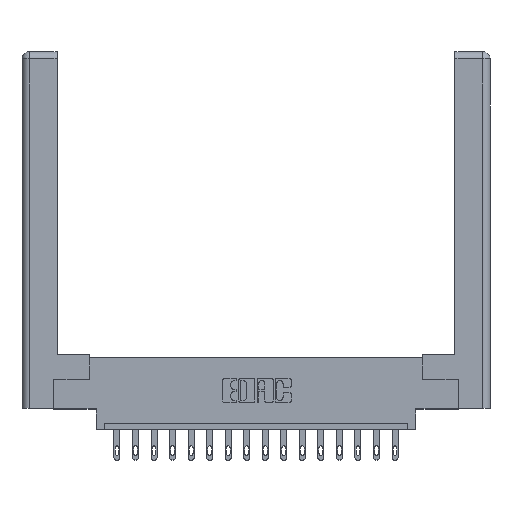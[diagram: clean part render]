
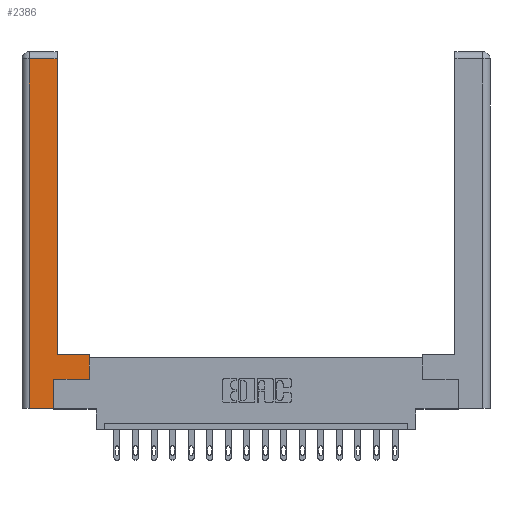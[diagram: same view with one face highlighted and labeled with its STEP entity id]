
A CAD part, top view. The second image highlights one B-rep face of the part: STEP entity #2386.
In plain terms, the highlighted planar face has unit normal (0, 0, 1).
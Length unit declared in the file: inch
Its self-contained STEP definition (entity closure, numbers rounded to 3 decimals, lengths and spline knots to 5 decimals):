
#383 = CARTESIAN_POINT ( 'NONE',  ( 0.565, 0.45, 0. ) ) ;
#586 = VERTEX_POINT ( 'NONE', #3452 ) ;
#649 = CARTESIAN_POINT ( 'NONE',  ( 0.265, 0.245, 0. ) ) ;
#767 = CARTESIAN_POINT ( 'NONE',  ( 0.265, 0.245, 0. ) ) ;
#811 = ORIENTED_EDGE ( 'NONE', *, *, #1996, .T. ) ;
#1185 = CARTESIAN_POINT ( 'NONE',  ( 0.0615, 2.94, 0. ) ) ;
#1255 = VERTEX_POINT ( 'NONE', #9296 ) ;
#1418 = LINE ( 'NONE', #2562, #4699 ) ;
#1996 = EDGE_CURVE ( 'NONE', #586, #2529, #3529, .T. ) ;
#2221 = EDGE_CURVE ( 'NONE', #3925, #12713, #11321, .T. ) ;
#2386 = ADVANCED_FACE ( 'NONE', ( #11115 ), #7721, .F. ) ;
#2529 = VERTEX_POINT ( 'NONE', #13905 ) ;
#2562 = CARTESIAN_POINT ( 'NONE',  ( 0.265, 0., 0. ) ) ;
#2714 = CARTESIAN_POINT ( 'NONE',  ( 0.295, 3., 0. ) ) ;
#2833 = VECTOR ( 'NONE', #14444, 39.37008 ) ;
#3452 = CARTESIAN_POINT ( 'NONE',  ( 0.565, 0.245, 0. ) ) ;
#3529 = LINE ( 'NONE', #383, #3743 ) ;
#3743 = VECTOR ( 'NONE', #8595, 39.37008 ) ;
#3925 = VERTEX_POINT ( 'NONE', #11253 ) ;
#4699 = VECTOR ( 'NONE', #16469, 39.37008 ) ;
#4761 = DIRECTION ( 'NONE',  ( 0., 0., -1. ) ) ;
#5223 = LINE ( 'NONE', #767, #2833 ) ;
#5252 = VECTOR ( 'NONE', #15096, 39.37008 ) ;
#5831 = CARTESIAN_POINT ( 'NONE',  ( 0.565, 0.245, 0. ) ) ;
#6447 = EDGE_LOOP ( 'NONE', ( #8512, #17109, #12081, #16028, #7685, #17517, #811, #10173 ) ) ;
#6789 = DIRECTION ( 'NONE',  ( -1., 0., 0. ) ) ;
#7070 = DIRECTION ( 'NONE',  ( 0., 1., 0. ) ) ;
#7476 = CARTESIAN_POINT ( 'NONE',  ( 0.295, 2.94, 0. ) ) ;
#7618 = CARTESIAN_POINT ( 'NONE',  ( 0.0615, 0., 0. ) ) ;
#7685 = ORIENTED_EDGE ( 'NONE', *, *, #9998, .T. ) ;
#7721 = PLANE ( 'NONE',  #12204 ) ;
#7992 = EDGE_CURVE ( 'NONE', #9952, #586, #13423, .T. ) ;
#8190 = VERTEX_POINT ( 'NONE', #7618 ) ;
#8512 = ORIENTED_EDGE ( 'NONE', *, *, #2221, .T. ) ;
#8595 = DIRECTION ( 'NONE',  ( 0., 1., 0. ) ) ;
#9296 = CARTESIAN_POINT ( 'NONE',  ( 0.0615, 2.94, 0. ) ) ;
#9835 = VECTOR ( 'NONE', #13062, 39.37008 ) ;
#9952 = VERTEX_POINT ( 'NONE', #649 ) ;
#9998 = EDGE_CURVE ( 'NONE', #17233, #9952, #5223, .T. ) ;
#10173 = ORIENTED_EDGE ( 'NONE', *, *, #10899, .T. ) ;
#10814 = VECTOR ( 'NONE', #11453, 39.37008 ) ;
#10899 = EDGE_CURVE ( 'NONE', #2529, #3925, #13513, .T. ) ;
#11115 = FACE_OUTER_BOUND ( 'NONE', #6447, .T. ) ;
#11253 = CARTESIAN_POINT ( 'NONE',  ( 0.295, 0.45, 0. ) ) ;
#11321 = LINE ( 'NONE', #2714, #14573 ) ;
#11329 = LINE ( 'NONE', #14396, #9835 ) ;
#11453 = DIRECTION ( 'NONE',  ( 1., 0., 0. ) ) ;
#11678 = EDGE_CURVE ( 'NONE', #1255, #8190, #11329, .T. ) ;
#11982 = EDGE_CURVE ( 'NONE', #12713, #1255, #16945, .T. ) ;
#12081 = ORIENTED_EDGE ( 'NONE', *, *, #11678, .T. ) ;
#12204 = AXIS2_PLACEMENT_3D ( 'NONE', #17143, #4761, #17206 ) ;
#12651 = VECTOR ( 'NONE', #6789, 39.37008 ) ;
#12713 = VERTEX_POINT ( 'NONE', #7476 ) ;
#13062 = DIRECTION ( 'NONE',  ( 0., -1., 0. ) ) ;
#13423 = LINE ( 'NONE', #5831, #10814 ) ;
#13513 = LINE ( 'NONE', #14958, #12651 ) ;
#13905 = CARTESIAN_POINT ( 'NONE',  ( 0.565, 0.45, 0. ) ) ;
#14396 = CARTESIAN_POINT ( 'NONE',  ( 0.0615, 0., 0. ) ) ;
#14444 = DIRECTION ( 'NONE',  ( 0., 1., 0. ) ) ;
#14573 = VECTOR ( 'NONE', #7070, 39.37008 ) ;
#14940 = EDGE_CURVE ( 'NONE', #8190, #17233, #1418, .T. ) ;
#14958 = CARTESIAN_POINT ( 'NONE',  ( 0.295, 0.45, 0. ) ) ;
#15096 = DIRECTION ( 'NONE',  ( -1., 0., 0. ) ) ;
#16028 = ORIENTED_EDGE ( 'NONE', *, *, #14940, .T. ) ;
#16469 = DIRECTION ( 'NONE',  ( 1., 0., 0. ) ) ;
#16719 = CARTESIAN_POINT ( 'NONE',  ( 0.265, 0., 0. ) ) ;
#16945 = LINE ( 'NONE', #1185, #5252 ) ;
#17109 = ORIENTED_EDGE ( 'NONE', *, *, #11982, .T. ) ;
#17143 = CARTESIAN_POINT ( 'NONE',  ( 0., 0., 0. ) ) ;
#17206 = DIRECTION ( 'NONE',  ( -1., 0., 0. ) ) ;
#17233 = VERTEX_POINT ( 'NONE', #16719 ) ;
#17517 = ORIENTED_EDGE ( 'NONE', *, *, #7992, .T. ) ;
